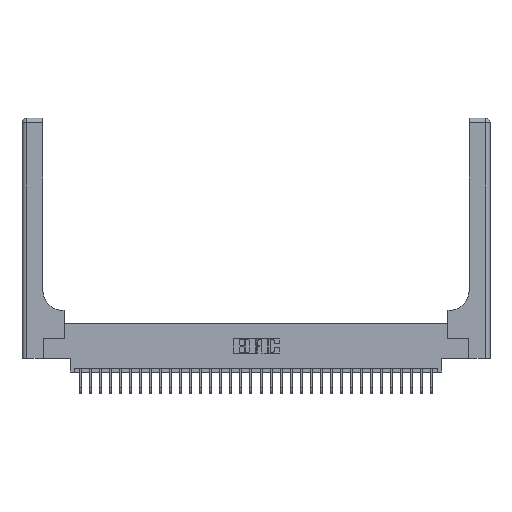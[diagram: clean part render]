
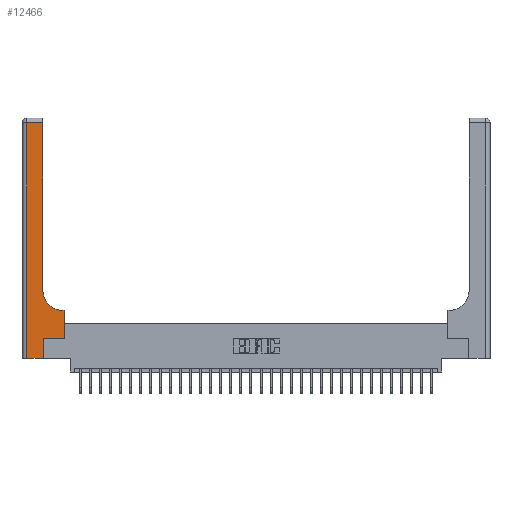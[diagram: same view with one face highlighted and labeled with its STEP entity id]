
A CAD part, top view. The second image highlights one B-rep face of the part: STEP entity #12466.
In plain terms, the highlighted planar face has unit normal (0, 0, 1).
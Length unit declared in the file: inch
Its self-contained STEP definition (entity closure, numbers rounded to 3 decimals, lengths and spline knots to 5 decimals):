
#358 = EDGE_LOOP ( 'NONE', ( #25066, #18202, #1269, #3749, #5156, #22432, #1019, #25169, #9378 ) ) ;
#1019 = ORIENTED_EDGE ( 'NONE', *, *, #19825, .T. ) ;
#1269 = ORIENTED_EDGE ( 'NONE', *, *, #20361, .T. ) ;
#2232 = CARTESIAN_POINT ( 'NONE',  ( 0.06, 0., 0.37 ) ) ;
#2654 = VERTEX_POINT ( 'NONE', #13744 ) ;
#3333 = CARTESIAN_POINT ( 'NONE',  ( 0.528, 0.25, 0.37 ) ) ;
#3397 = PLANE ( 'NONE',  #20211 ) ;
#3749 = ORIENTED_EDGE ( 'NONE', *, *, #23117, .T. ) ;
#5019 = EDGE_CURVE ( 'NONE', #20633, #6931, #27960, .T. ) ;
#5156 = ORIENTED_EDGE ( 'NONE', *, *, #8390, .T. ) ;
#6082 = CARTESIAN_POINT ( 'NONE',  ( 0.26, 0.6, 0.37 ) ) ;
#6126 = VERTEX_POINT ( 'NONE', #14702 ) ;
#6439 = DIRECTION ( 'NONE',  ( 1., 0., 0. ) ) ;
#6931 = VERTEX_POINT ( 'NONE', #26593 ) ;
#6966 = VECTOR ( 'NONE', #22608, 39.37008 ) ;
#7875 = CARTESIAN_POINT ( 'NONE',  ( 0.265, 0., 0.37 ) ) ;
#7881 = LINE ( 'NONE', #7875, #24731 ) ;
#7895 = DIRECTION ( 'NONE',  ( -1., 0., 0. ) ) ;
#7951 = CARTESIAN_POINT ( 'NONE',  ( 0.265, 0., 0.37 ) ) ;
#8390 = EDGE_CURVE ( 'NONE', #16128, #18503, #7881, .T. ) ;
#9092 = VECTOR ( 'NONE', #6439, 39.37008 ) ;
#9185 = DIRECTION ( 'NONE',  ( 1., 0., 0. ) ) ;
#9378 = ORIENTED_EDGE ( 'NONE', *, *, #17876, .T. ) ;
#9432 = CARTESIAN_POINT ( 'NONE',  ( 0.06, 3., 0.37 ) ) ;
#10064 = DIRECTION ( 'NONE',  ( 0., 1., 0. ) ) ;
#10161 = LINE ( 'NONE', #25403, #21179 ) ;
#10293 = VECTOR ( 'NONE', #19321, 39.37008 ) ;
#10786 = VECTOR ( 'NONE', #9185, 39.37008 ) ;
#11767 = LINE ( 'NONE', #25944, #10293 ) ;
#12270 = DIRECTION ( 'NONE',  ( -1., 0., 0. ) ) ;
#12338 = VERTEX_POINT ( 'NONE', #2232 ) ;
#12466 = ADVANCED_FACE ( 'NONE', ( #18839 ), #3397, .F. ) ;
#12490 = DIRECTION ( 'NONE',  ( 0., 0., -1. ) ) ;
#13744 = CARTESIAN_POINT ( 'NONE',  ( 0.06, 2.94, 0.37 ) ) ;
#13760 = EDGE_CURVE ( 'NONE', #6126, #2654, #10161, .T. ) ;
#14430 = CARTESIAN_POINT ( 'NONE',  ( 0., 3., 0.37 ) ) ;
#14450 = EDGE_CURVE ( 'NONE', #18503, #25995, #14967, .T. ) ;
#14702 = CARTESIAN_POINT ( 'NONE',  ( 0.26, 2.94, 0.37 ) ) ;
#14937 = AXIS2_PLACEMENT_3D ( 'NONE', #25615, #12490, #27840 ) ;
#14967 = LINE ( 'NONE', #17404, #9092 ) ;
#15834 = CARTESIAN_POINT ( 'NONE',  ( 0., 0., 0.37 ) ) ;
#16128 = VERTEX_POINT ( 'NONE', #7951 ) ;
#16273 = VECTOR ( 'NONE', #25877, 39.37008 ) ;
#17404 = CARTESIAN_POINT ( 'NONE',  ( 0.265, 0.25, 0.37 ) ) ;
#17755 = VERTEX_POINT ( 'NONE', #18612 ) ;
#17876 = EDGE_CURVE ( 'NONE', #6931, #17755, #20475, .T. ) ;
#18202 = ORIENTED_EDGE ( 'NONE', *, *, #13760, .T. ) ;
#18503 = VERTEX_POINT ( 'NONE', #18649 ) ;
#18612 = CARTESIAN_POINT ( 'NONE',  ( 0.26, 0.85, 0.37 ) ) ;
#18649 = CARTESIAN_POINT ( 'NONE',  ( 0.265, 0.25, 0.37 ) ) ;
#18668 = VECTOR ( 'NONE', #20989, 39.37008 ) ;
#18839 = FACE_OUTER_BOUND ( 'NONE', #358, .T. ) ;
#19321 = DIRECTION ( 'NONE',  ( 0., 1., 0. ) ) ;
#19522 = CARTESIAN_POINT ( 'NONE',  ( 0.528, 0.6, 0.37 ) ) ;
#19825 = EDGE_CURVE ( 'NONE', #25995, #20633, #25197, .T. ) ;
#20211 = AXIS2_PLACEMENT_3D ( 'NONE', #14430, #21053, #7895 ) ;
#20361 = EDGE_CURVE ( 'NONE', #2654, #12338, #23111, .T. ) ;
#20475 = CIRCLE ( 'NONE', #14937, 0.25 ) ;
#20579 = EDGE_CURVE ( 'NONE', #17755, #6126, #11767, .T. ) ;
#20633 = VERTEX_POINT ( 'NONE', #19522 ) ;
#20989 = DIRECTION ( 'NONE',  ( 0., 1., 0. ) ) ;
#21053 = DIRECTION ( 'NONE',  ( 0., 0., -1. ) ) ;
#21179 = VECTOR ( 'NONE', #12270, 39.37008 ) ;
#22432 = ORIENTED_EDGE ( 'NONE', *, *, #14450, .T. ) ;
#22608 = DIRECTION ( 'NONE',  ( 0., -1., 0. ) ) ;
#23111 = LINE ( 'NONE', #9432, #6966 ) ;
#23117 = EDGE_CURVE ( 'NONE', #12338, #16128, #27610, .T. ) ;
#24731 = VECTOR ( 'NONE', #10064, 39.37008 ) ;
#25065 = CARTESIAN_POINT ( 'NONE',  ( 0.528, 0.25, 0.37 ) ) ;
#25066 = ORIENTED_EDGE ( 'NONE', *, *, #20579, .T. ) ;
#25169 = ORIENTED_EDGE ( 'NONE', *, *, #5019, .T. ) ;
#25197 = LINE ( 'NONE', #3333, #18668 ) ;
#25403 = CARTESIAN_POINT ( 'NONE',  ( 0., 2.94, 0.37 ) ) ;
#25615 = CARTESIAN_POINT ( 'NONE',  ( 0.51, 0.85, 0.37 ) ) ;
#25877 = DIRECTION ( 'NONE',  ( -1., 0., 0. ) ) ;
#25944 = CARTESIAN_POINT ( 'NONE',  ( 0.26, 3., 0.37 ) ) ;
#25995 = VERTEX_POINT ( 'NONE', #25065 ) ;
#26593 = CARTESIAN_POINT ( 'NONE',  ( 0.51, 0.6, 0.37 ) ) ;
#27610 = LINE ( 'NONE', #15834, #10786 ) ;
#27840 = DIRECTION ( 'NONE',  ( 1., 0., 0. ) ) ;
#27960 = LINE ( 'NONE', #6082, #16273 ) ;
